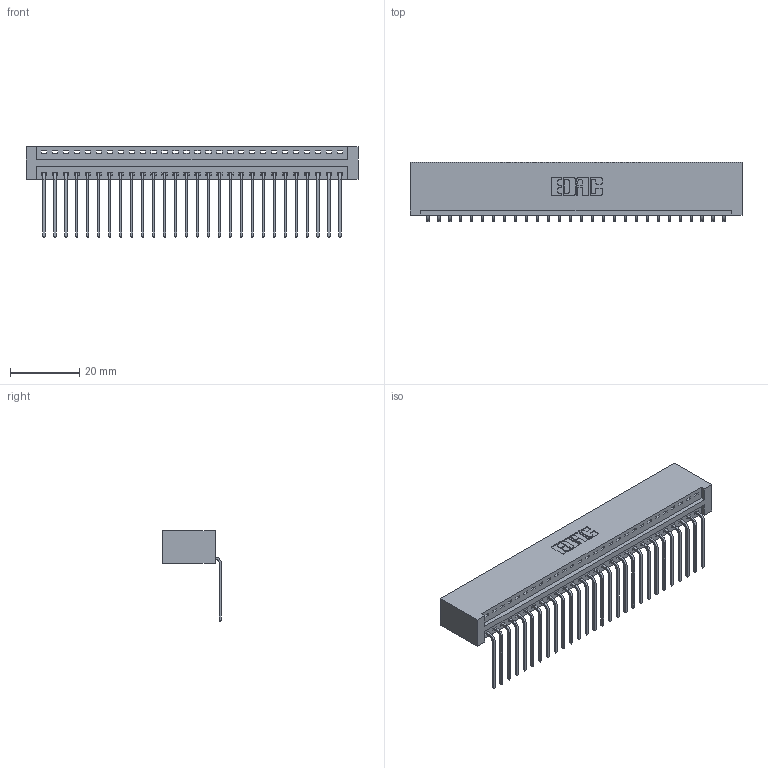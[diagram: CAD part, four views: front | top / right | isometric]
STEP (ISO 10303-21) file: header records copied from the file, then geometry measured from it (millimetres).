
FILE_DESCRIPTION (( 'STEP AP203' ), '1' );
FILE_NAME ('346-028-559-101.STEP', '2018-08-22T02:32:52', ( '' ), ( '' ), 'SwSTEP 2.0', 'SolidWorks 2016', '' );
FILE_SCHEMA (( 'CONFIG_CONTROL_DESIGN' ));
Length unit declared in the file: inch
Products named in the file (3): 346 Part_No Mounting Lugs; 345-292-001_558 559 Tail - 1; 346-028-559-101
Assembly tree (29 placements, depth 2):
  346-028-559-101
    346 Part_No Mounting Lugs
    345-292-001_558 559 Tail - 1  x28
Bounding box: 96.14 x 17.08 x 26.16 mm (x, y, z)
Volume: 9748.9 mm3; surface area: 12665.4 mm2
Topology: 29 solids, 29 shells, 1794 faces, 5401 edges, 3562 vertices
Faces by surface type: plane 1248, cylinder 546
Entity records: 19069 total; most frequent: CARTESIAN_POINT 3280, ORIENTED_EDGE 3242, DIRECTION 2905, EDGE_CURVE 1621, LINE 1385, VECTOR 1385, VERTEX_POINT 1078, AXIS2_PLACEMENT_3D 760
